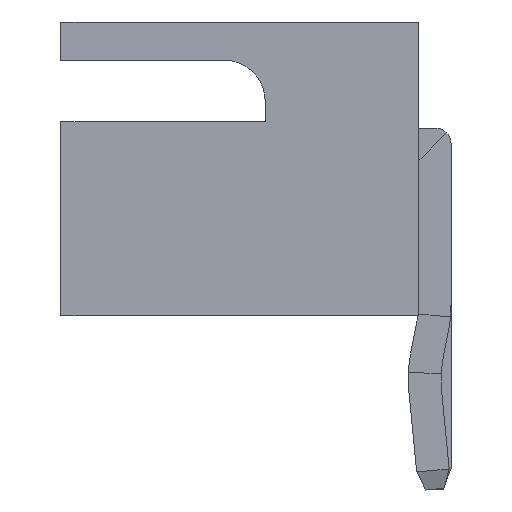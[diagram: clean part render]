
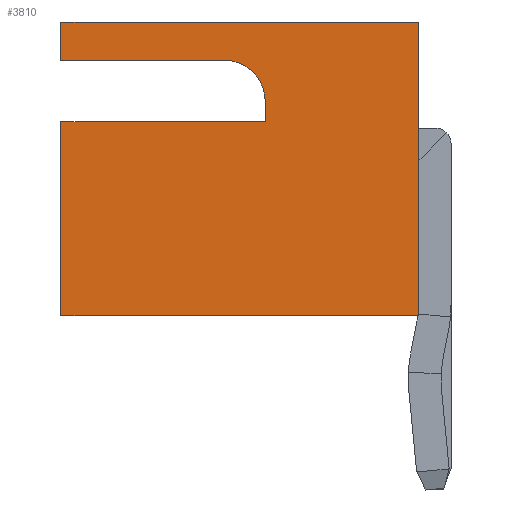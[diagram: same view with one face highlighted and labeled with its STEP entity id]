
A CAD part, left-side view. The second image highlights one B-rep face of the part: STEP entity #3810.
In plain terms, the highlighted planar face has unit normal (-1, 0, 0).
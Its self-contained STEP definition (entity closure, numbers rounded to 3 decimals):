
#7 = CARTESIAN_POINT ( 'NONE',  ( -6.25, 3.8, 2.125 ) ) ;
#61 = VECTOR ( 'NONE', #1590, 1000. ) ;
#72 = LINE ( 'NONE', #842, #425 ) ;
#100 = EDGE_CURVE ( 'NONE', #3219, #4019, #880, .T. ) ;
#118 = VERTEX_POINT ( 'NONE', #3123 ) ;
#216 = VERTEX_POINT ( 'NONE', #4370 ) ;
#246 = EDGE_CURVE ( 'NONE', #3335, #4019, #4343, .T. ) ;
#425 = VECTOR ( 'NONE', #2652, 1000. ) ;
#583 = CARTESIAN_POINT ( 'NONE',  ( -6.25, 3., 1.325 ) ) ;
#651 = ORIENTED_EDGE ( 'NONE', *, *, #246, .F. ) ;
#662 = CARTESIAN_POINT ( 'NONE',  ( -6.25, 3., 0.925 ) ) ;
#667 = EDGE_CURVE ( 'NONE', #3356, #2325, #933, .T. ) ;
#678 = CARTESIAN_POINT ( 'NONE',  ( -6.25, 7., 2.125 ) ) ;
#688 = ORIENTED_EDGE ( 'NONE', *, *, #2049, .F. ) ;
#723 = CARTESIAN_POINT ( 'NONE',  ( -6.25, 7., -2.875 ) ) ;
#755 = CARTESIAN_POINT ( 'NONE',  ( -6.25, 3.8, 1.325 ) ) ;
#762 = VECTOR ( 'NONE', #3857, 1000. ) ;
#842 = CARTESIAN_POINT ( 'NONE',  ( -6.25, 7., 0.925 ) ) ;
#880 = LINE ( 'NONE', #1637, #762 ) ;
#933 = CIRCLE ( 'NONE', #3739, 0.8 ) ;
#963 = EDGE_CURVE ( 'NONE', #118, #2835, #3844, .T. ) ;
#972 = DIRECTION ( 'NONE',  ( 0., -1., 0. ) ) ;
#989 = LINE ( 'NONE', #3589, #1920 ) ;
#1109 = DIRECTION ( 'NONE',  ( 1., 0., 0. ) ) ;
#1495 = DIRECTION ( 'NONE',  ( 0., -1., 0. ) ) ;
#1590 = DIRECTION ( 'NONE',  ( 0., 0., 1. ) ) ;
#1637 = CARTESIAN_POINT ( 'NONE',  ( -6.25, 0., -2.875 ) ) ;
#1685 = VECTOR ( 'NONE', #1495, 1000. ) ;
#1821 = FACE_OUTER_BOUND ( 'NONE', #2799, .T. ) ;
#1827 = LINE ( 'NONE', #723, #3863 ) ;
#1840 = ORIENTED_EDGE ( 'NONE', *, *, #2410, .T. ) ;
#1864 = CARTESIAN_POINT ( 'NONE',  ( -6.25, 3., 1.325 ) ) ;
#1913 = DIRECTION ( 'NONE',  ( 0., 0., -1. ) ) ;
#1920 = VECTOR ( 'NONE', #2444, 1000. ) ;
#1933 = ORIENTED_EDGE ( 'NONE', *, *, #963, .F. ) ;
#2049 = EDGE_CURVE ( 'NONE', #216, #3335, #1827, .T. ) ;
#2325 = VERTEX_POINT ( 'NONE', #583 ) ;
#2410 = EDGE_CURVE ( 'NONE', #2325, #2690, #3992, .T. ) ;
#2432 = EDGE_CURVE ( 'NONE', #216, #3356, #4473, .T. ) ;
#2444 = DIRECTION ( 'NONE',  ( 0., -1., 0. ) ) ;
#2456 = CARTESIAN_POINT ( 'NONE',  ( -6.25, 0., -2.875 ) ) ;
#2574 = ORIENTED_EDGE ( 'NONE', *, *, #3923, .T. ) ;
#2606 = DIRECTION ( 'NONE',  ( 0., 0., -1. ) ) ;
#2621 = DIRECTION ( 'NONE',  ( 1., 0., 0. ) ) ;
#2652 = DIRECTION ( 'NONE',  ( 0., 1., 0. ) ) ;
#2690 = VERTEX_POINT ( 'NONE', #662 ) ;
#2799 = EDGE_LOOP ( 'NONE', ( #688, #3023, #3199, #1840, #2574, #1933, #4197, #3668, #651 ) ) ;
#2835 = VERTEX_POINT ( 'NONE', #2947 ) ;
#2947 = CARTESIAN_POINT ( 'NONE',  ( -6.25, 7., 0.925 ) ) ;
#3023 = ORIENTED_EDGE ( 'NONE', *, *, #2432, .T. ) ;
#3123 = CARTESIAN_POINT ( 'NONE',  ( -6.25, 7., -2.875 ) ) ;
#3186 = CARTESIAN_POINT ( 'NONE',  ( -6.25, 0., 2.875 ) ) ;
#3199 = ORIENTED_EDGE ( 'NONE', *, *, #667, .T. ) ;
#3219 = VERTEX_POINT ( 'NONE', #2456 ) ;
#3335 = VERTEX_POINT ( 'NONE', #4392 ) ;
#3356 = VERTEX_POINT ( 'NONE', #7 ) ;
#3465 = CARTESIAN_POINT ( 'NONE',  ( -6.25, 7., -2.875 ) ) ;
#3485 = AXIS2_PLACEMENT_3D ( 'NONE', #4458, #1109, #2606 ) ;
#3589 = CARTESIAN_POINT ( 'NONE',  ( -6.25, 7., -2.875 ) ) ;
#3642 = CARTESIAN_POINT ( 'NONE',  ( -6.25, 7., 2.875 ) ) ;
#3668 = ORIENTED_EDGE ( 'NONE', *, *, #100, .T. ) ;
#3697 = PLANE ( 'NONE',  #3485 ) ;
#3739 = AXIS2_PLACEMENT_3D ( 'NONE', #755, #2621, #4072 ) ;
#3787 = VECTOR ( 'NONE', #1913, 1000. ) ;
#3810 = ADVANCED_FACE ( 'NONE', ( #1821 ), #3697, .F. ) ;
#3844 = LINE ( 'NONE', #3465, #61 ) ;
#3857 = DIRECTION ( 'NONE',  ( 0., 0., 1. ) ) ;
#3863 = VECTOR ( 'NONE', #4390, 1000. ) ;
#3923 = EDGE_CURVE ( 'NONE', #2690, #2835, #72, .T. ) ;
#3992 = LINE ( 'NONE', #1864, #3787 ) ;
#4019 = VERTEX_POINT ( 'NONE', #3186 ) ;
#4072 = DIRECTION ( 'NONE',  ( 0., 0., -1. ) ) ;
#4136 = EDGE_CURVE ( 'NONE', #118, #3219, #989, .T. ) ;
#4197 = ORIENTED_EDGE ( 'NONE', *, *, #4136, .T. ) ;
#4343 = LINE ( 'NONE', #3642, #4511 ) ;
#4370 = CARTESIAN_POINT ( 'NONE',  ( -6.25, 7., 2.125 ) ) ;
#4390 = DIRECTION ( 'NONE',  ( 0., 0., 1. ) ) ;
#4392 = CARTESIAN_POINT ( 'NONE',  ( -6.25, 7., 2.875 ) ) ;
#4458 = CARTESIAN_POINT ( 'NONE',  ( -6.25, 7., -2.875 ) ) ;
#4473 = LINE ( 'NONE', #678, #1685 ) ;
#4511 = VECTOR ( 'NONE', #972, 1000. ) ;
